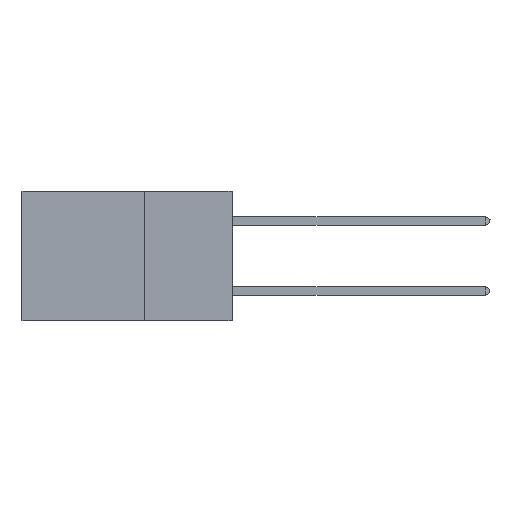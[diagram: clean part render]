
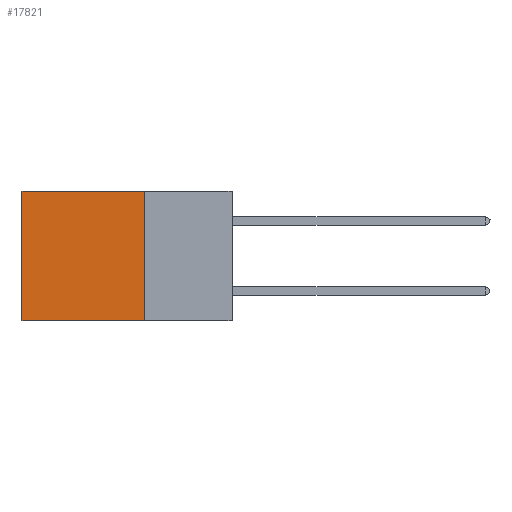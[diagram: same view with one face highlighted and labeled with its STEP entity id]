
A CAD part, left-side view. The second image highlights one B-rep face of the part: STEP entity #17821.
In plain terms, the highlighted planar face has unit normal (-1, 0, 0).
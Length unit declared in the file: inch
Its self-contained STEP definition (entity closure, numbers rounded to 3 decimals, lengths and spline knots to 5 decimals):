
#217 = DIRECTION ( 'NONE',  ( 0., 0., -1. ) ) ;
#544 = VERTEX_POINT ( 'NONE', #13518 ) ;
#927 = ORIENTED_EDGE ( 'NONE', *, *, #5137, .F. ) ;
#2479 = CARTESIAN_POINT ( 'NONE',  ( 0.2875, 0.25, -0.37 ) ) ;
#3223 = LINE ( 'NONE', #17116, #7748 ) ;
#3265 = AXIS2_PLACEMENT_3D ( 'NONE', #15835, #17393, #8154 ) ;
#3942 = VERTEX_POINT ( 'NONE', #12437 ) ;
#4035 = VECTOR ( 'NONE', #15148, 39.37008 ) ;
#4054 = EDGE_LOOP ( 'NONE', ( #5672, #14611, #927, #5102 ) ) ;
#5102 = ORIENTED_EDGE ( 'NONE', *, *, #7853, .T. ) ;
#5137 = EDGE_CURVE ( 'NONE', #9728, #3942, #10703, .T. ) ;
#5416 = VECTOR ( 'NONE', #13286, 39.37008 ) ;
#5672 = ORIENTED_EDGE ( 'NONE', *, *, #10121, .T. ) ;
#5761 = CARTESIAN_POINT ( 'NONE',  ( 0.2875, 0.25, 0. ) ) ;
#6170 = VERTEX_POINT ( 'NONE', #16641 ) ;
#6370 = LINE ( 'NONE', #2479, #5416 ) ;
#7127 = VECTOR ( 'NONE', #15803, 39.37008 ) ;
#7609 = LINE ( 'NONE', #5761, #4035 ) ;
#7748 = VECTOR ( 'NONE', #217, 39.37008 ) ;
#7853 = EDGE_CURVE ( 'NONE', #9728, #544, #7609, .T. ) ;
#8154 = DIRECTION ( 'NONE',  ( 0., 0., -1. ) ) ;
#9728 = VERTEX_POINT ( 'NONE', #12626 ) ;
#10121 = EDGE_CURVE ( 'NONE', #544, #6170, #3223, .T. ) ;
#10703 = LINE ( 'NONE', #17156, #7127 ) ;
#12437 = CARTESIAN_POINT ( 'NONE',  ( 0.2875, 0.25, -0.37 ) ) ;
#12626 = CARTESIAN_POINT ( 'NONE',  ( 0.2875, 0.25, 0. ) ) ;
#13286 = DIRECTION ( 'NONE',  ( 0., 1., 0. ) ) ;
#13518 = CARTESIAN_POINT ( 'NONE',  ( 0.2875, 0.6, 0. ) ) ;
#14192 = EDGE_CURVE ( 'NONE', #3942, #6170, #6370, .T. ) ;
#14611 = ORIENTED_EDGE ( 'NONE', *, *, #14192, .F. ) ;
#15148 = DIRECTION ( 'NONE',  ( 0., 1., 0. ) ) ;
#15803 = DIRECTION ( 'NONE',  ( 0., 0., -1. ) ) ;
#15835 = CARTESIAN_POINT ( 'NONE',  ( 0.2875, 0.25, 0. ) ) ;
#15898 = PLANE ( 'NONE',  #3265 ) ;
#16641 = CARTESIAN_POINT ( 'NONE',  ( 0.2875, 0.6, -0.37 ) ) ;
#17116 = CARTESIAN_POINT ( 'NONE',  ( 0.2875, 0.6, 0. ) ) ;
#17156 = CARTESIAN_POINT ( 'NONE',  ( 0.2875, 0.25, 0. ) ) ;
#17393 = DIRECTION ( 'NONE',  ( 1., 0., 0. ) ) ;
#17821 = ADVANCED_FACE ( 'NONE', ( #17831 ), #15898, .F. ) ;
#17831 = FACE_OUTER_BOUND ( 'NONE', #4054, .T. ) ;
